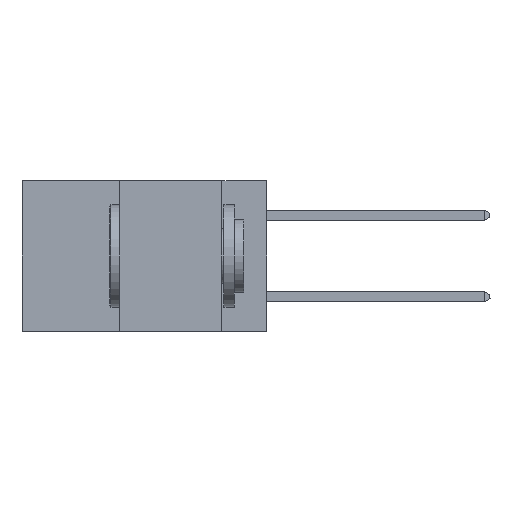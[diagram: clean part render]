
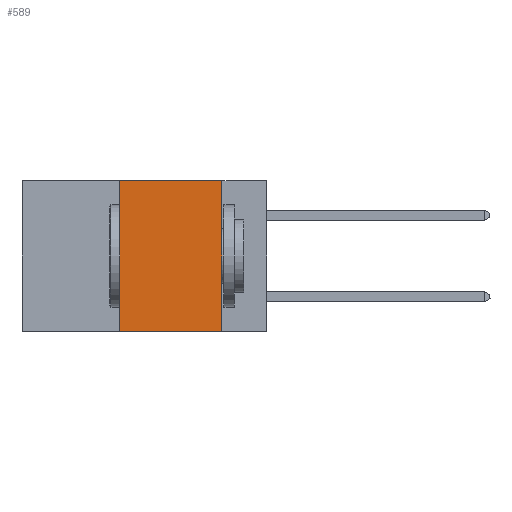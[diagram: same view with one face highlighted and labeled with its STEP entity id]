
A CAD part, left-side view. The second image highlights one B-rep face of the part: STEP entity #589.
In plain terms, the highlighted planar face has unit normal (-1, 0, 0).
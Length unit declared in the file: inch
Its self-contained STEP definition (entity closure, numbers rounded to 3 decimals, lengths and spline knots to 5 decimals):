
#589 = ADVANCED_FACE ( 'NONE', ( #7081 ), #24009, .F. ) ;
#1500 = VECTOR ( 'NONE', #14678, 39.37008 ) ;
#2345 = CARTESIAN_POINT ( 'NONE',  ( 0., 0.36, 0. ) ) ;
#4190 = CARTESIAN_POINT ( 'NONE',  ( 0., 0.11, 0. ) ) ;
#5021 = EDGE_CURVE ( 'NONE', #28950, #26435, #19868, .T. ) ;
#5428 = AXIS2_PLACEMENT_3D ( 'NONE', #24155, #23855, #23762 ) ;
#7081 = FACE_OUTER_BOUND ( 'NONE', #21433, .T. ) ;
#7340 = CARTESIAN_POINT ( 'NONE',  ( 0., 0.36, 0. ) ) ;
#7691 = CARTESIAN_POINT ( 'NONE',  ( 0., 0.36, -0.37 ) ) ;
#8124 = VERTEX_POINT ( 'NONE', #7691 ) ;
#10958 = DIRECTION ( 'NONE',  ( 0., 0., -1. ) ) ;
#11300 = ORIENTED_EDGE ( 'NONE', *, *, #12316, .T. ) ;
#12316 = EDGE_CURVE ( 'NONE', #8124, #27462, #13481, .T. ) ;
#12468 = CARTESIAN_POINT ( 'NONE',  ( 0., 0.6, -0.37 ) ) ;
#13020 = ORIENTED_EDGE ( 'NONE', *, *, #15281, .F. ) ;
#13481 = LINE ( 'NONE', #12468, #1500 ) ;
#14678 = DIRECTION ( 'NONE',  ( 0., -1., 0. ) ) ;
#15052 = LINE ( 'NONE', #4190, #20395 ) ;
#15108 = EDGE_CURVE ( 'NONE', #26435, #27462, #15052, .T. ) ;
#15256 = CARTESIAN_POINT ( 'NONE',  ( 0., 0.11, 0. ) ) ;
#15281 = EDGE_CURVE ( 'NONE', #8124, #28950, #23518, .T. ) ;
#16187 = DIRECTION ( 'NONE',  ( 0., 0., 1. ) ) ;
#18451 = VECTOR ( 'NONE', #28383, 39.37008 ) ;
#19868 = LINE ( 'NONE', #28478, #18451 ) ;
#20395 = VECTOR ( 'NONE', #10958, 39.37008 ) ;
#21433 = EDGE_LOOP ( 'NONE', ( #24645, #23581, #13020, #11300 ) ) ;
#22825 = VECTOR ( 'NONE', #16187, 39.37008 ) ;
#23518 = LINE ( 'NONE', #7340, #22825 ) ;
#23581 = ORIENTED_EDGE ( 'NONE', *, *, #5021, .F. ) ;
#23762 = DIRECTION ( 'NONE',  ( 0., 0., -1. ) ) ;
#23855 = DIRECTION ( 'NONE',  ( 1., 0., 0. ) ) ;
#24009 = PLANE ( 'NONE',  #5428 ) ;
#24055 = CARTESIAN_POINT ( 'NONE',  ( 0., 0.11, -0.37 ) ) ;
#24155 = CARTESIAN_POINT ( 'NONE',  ( 0., 0.6, 0. ) ) ;
#24645 = ORIENTED_EDGE ( 'NONE', *, *, #15108, .F. ) ;
#26435 = VERTEX_POINT ( 'NONE', #15256 ) ;
#27462 = VERTEX_POINT ( 'NONE', #24055 ) ;
#28383 = DIRECTION ( 'NONE',  ( 0., -1., 0. ) ) ;
#28478 = CARTESIAN_POINT ( 'NONE',  ( 0., 0.6, 0. ) ) ;
#28950 = VERTEX_POINT ( 'NONE', #2345 ) ;
